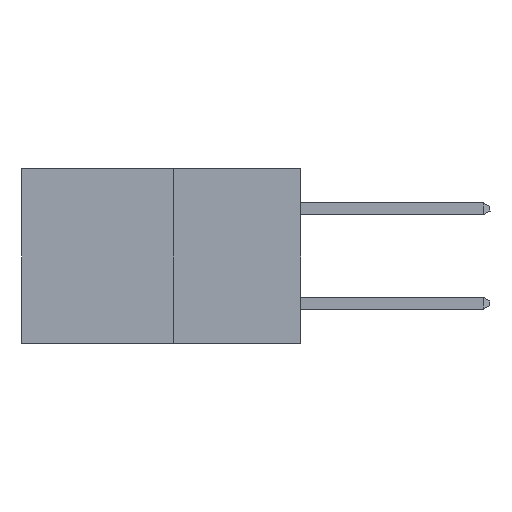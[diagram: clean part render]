
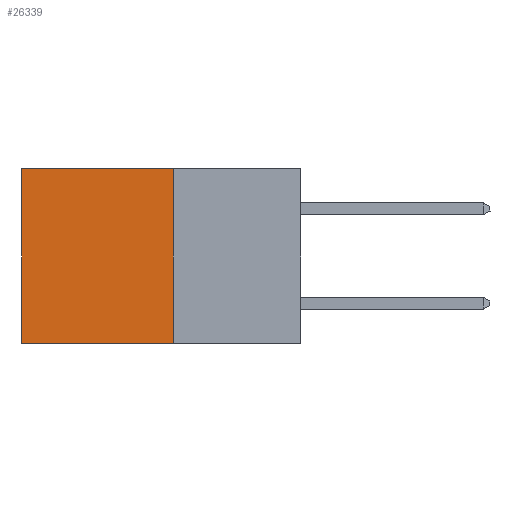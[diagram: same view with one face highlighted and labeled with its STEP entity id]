
A CAD part, left-side view. The second image highlights one B-rep face of the part: STEP entity #26339.
In plain terms, the highlighted planar face has unit normal (-1, 0, 0).
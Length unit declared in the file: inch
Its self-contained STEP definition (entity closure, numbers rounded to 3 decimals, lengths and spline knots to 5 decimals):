
#99 = PLANE ( 'NONE',  #12409 ) ;
#427 = EDGE_CURVE ( 'NONE', #9960, #16426, #23655, .T. ) ;
#689 = VECTOR ( 'NONE', #26656, 39.37008 ) ;
#1578 = CARTESIAN_POINT ( 'NONE',  ( 0.277, 0.27, -0.37 ) ) ;
#2333 = DIRECTION ( 'NONE',  ( 0., 0., -1. ) ) ;
#3626 = CARTESIAN_POINT ( 'NONE',  ( 0.277, 0.27, 0. ) ) ;
#3816 = VERTEX_POINT ( 'NONE', #23233 ) ;
#3937 = VECTOR ( 'NONE', #5778, 39.37008 ) ;
#5580 = ORIENTED_EDGE ( 'NONE', *, *, #10905, .T. ) ;
#5778 = DIRECTION ( 'NONE',  ( 0., 1., 0. ) ) ;
#9960 = VERTEX_POINT ( 'NONE', #1578 ) ;
#10763 = FACE_OUTER_BOUND ( 'NONE', #18291, .T. ) ;
#10905 = EDGE_CURVE ( 'NONE', #11793, #16426, #26874, .T. ) ;
#10987 = LINE ( 'NONE', #21412, #21336 ) ;
#11793 = VERTEX_POINT ( 'NONE', #24181 ) ;
#12409 = AXIS2_PLACEMENT_3D ( 'NONE', #21091, #14951, #2333 ) ;
#12733 = CARTESIAN_POINT ( 'NONE',  ( 0.277, 0.59, -0.37 ) ) ;
#14381 = ORIENTED_EDGE ( 'NONE', *, *, #21666, .F. ) ;
#14925 = DIRECTION ( 'NONE',  ( 0., 0., -1. ) ) ;
#14951 = DIRECTION ( 'NONE',  ( 1., 0., 0. ) ) ;
#15153 = ORIENTED_EDGE ( 'NONE', *, *, #23916, .T. ) ;
#15955 = VECTOR ( 'NONE', #14925, 39.37008 ) ;
#16426 = VERTEX_POINT ( 'NONE', #12733 ) ;
#18291 = EDGE_LOOP ( 'NONE', ( #5580, #24960, #14381, #15153 ) ) ;
#20581 = LINE ( 'NONE', #3626, #3937 ) ;
#21066 = CARTESIAN_POINT ( 'NONE',  ( 0.277, 0.59, -0.37 ) ) ;
#21091 = CARTESIAN_POINT ( 'NONE',  ( 0.277, 0.27, -0.37 ) ) ;
#21336 = VECTOR ( 'NONE', #23486, 39.37008 ) ;
#21412 = CARTESIAN_POINT ( 'NONE',  ( 0.277, 0.27, -0.37 ) ) ;
#21666 = EDGE_CURVE ( 'NONE', #3816, #9960, #10987, .T. ) ;
#23233 = CARTESIAN_POINT ( 'NONE',  ( 0.277, 0.27, 0. ) ) ;
#23486 = DIRECTION ( 'NONE',  ( 0., 0., -1. ) ) ;
#23655 = LINE ( 'NONE', #26563, #689 ) ;
#23916 = EDGE_CURVE ( 'NONE', #3816, #11793, #20581, .T. ) ;
#24181 = CARTESIAN_POINT ( 'NONE',  ( 0.277, 0.59, 0. ) ) ;
#24960 = ORIENTED_EDGE ( 'NONE', *, *, #427, .F. ) ;
#26339 = ADVANCED_FACE ( 'NONE', ( #10763 ), #99, .F. ) ;
#26563 = CARTESIAN_POINT ( 'NONE',  ( 0.277, 0.27, -0.37 ) ) ;
#26656 = DIRECTION ( 'NONE',  ( 0., 1., 0. ) ) ;
#26874 = LINE ( 'NONE', #21066, #15955 ) ;
